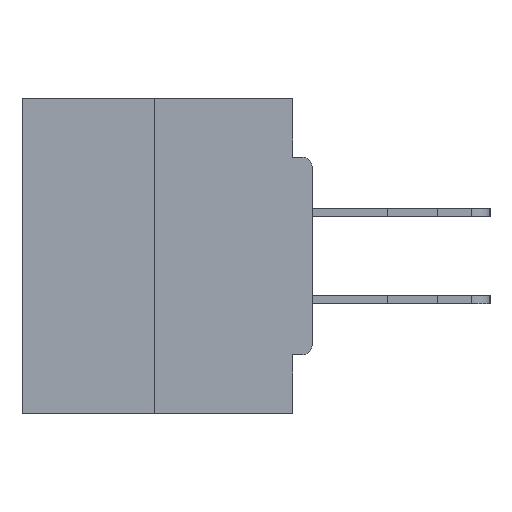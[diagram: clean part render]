
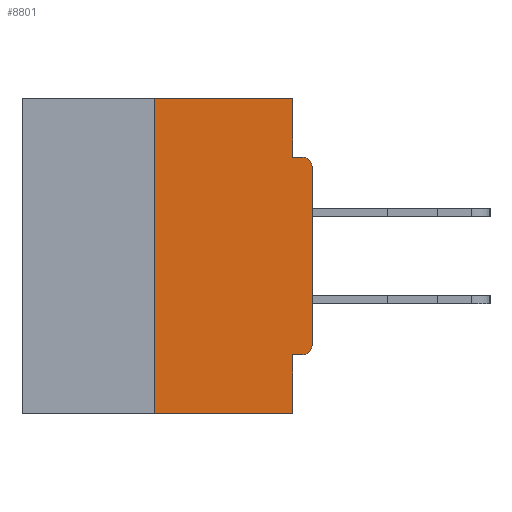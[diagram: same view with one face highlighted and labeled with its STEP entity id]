
A CAD part, left-side view. The second image highlights one B-rep face of the part: STEP entity #8801.
In plain terms, the highlighted planar face has unit normal (-1, 0, 0).
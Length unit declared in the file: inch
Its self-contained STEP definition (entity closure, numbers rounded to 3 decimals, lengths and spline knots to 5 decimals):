
#310 = CARTESIAN_POINT ( 'NONE',  ( 0., 0., -0.1085 ) ) ;
#431 = VERTEX_POINT ( 'NONE', #29109 ) ;
#497 = DIRECTION ( 'NONE',  ( 0., 0., -1. ) ) ;
#1847 = VECTOR ( 'NONE', #18469, 39.37008 ) ;
#2375 = EDGE_LOOP ( 'NONE', ( #6057, #5603, #20990, #12456, #24337, #6280, #20791, #26790, #5908, #17580 ) ) ;
#2600 = PLANE ( 'NONE',  #28627 ) ;
#3042 = VERTEX_POINT ( 'NONE', #310 ) ;
#3046 = EDGE_CURVE ( 'NONE', #3042, #20234, #15409, .T. ) ;
#3607 = DIRECTION ( 'NONE',  ( -1., 0., 0. ) ) ;
#3684 = CARTESIAN_POINT ( 'NONE',  ( 0., 0.015, -0.4065 ) ) ;
#3740 = CARTESIAN_POINT ( 'NONE',  ( 0., 0.46, 0. ) ) ;
#4171 = CARTESIAN_POINT ( 'NONE',  ( 0., 0.031, -0.0935 ) ) ;
#4238 = CARTESIAN_POINT ( 'NONE',  ( 0., 0.25, -0.5 ) ) ;
#4632 = CARTESIAN_POINT ( 'NONE',  ( 0., 0., 0. ) ) ;
#4866 = AXIS2_PLACEMENT_3D ( 'NONE', #27435, #3607, #22065 ) ;
#4919 = VECTOR ( 'NONE', #14685, 39.37008 ) ;
#5404 = EDGE_CURVE ( 'NONE', #27417, #28731, #22710, .T. ) ;
#5603 = ORIENTED_EDGE ( 'NONE', *, *, #30233, .F. ) ;
#5655 = DIRECTION ( 'NONE',  ( 0., -1., 0. ) ) ;
#5908 = ORIENTED_EDGE ( 'NONE', *, *, #34198, .F. ) ;
#6057 = ORIENTED_EDGE ( 'NONE', *, *, #5404, .F. ) ;
#6280 = ORIENTED_EDGE ( 'NONE', *, *, #24998, .T. ) ;
#6614 = DIRECTION ( 'NONE',  ( 0., -1., 0. ) ) ;
#7896 = EDGE_CURVE ( 'NONE', #29916, #29192, #21780, .T. ) ;
#8348 = CARTESIAN_POINT ( 'NONE',  ( 0., 0.25, 0. ) ) ;
#8578 = CIRCLE ( 'NONE', #30166, 0.015 ) ;
#8801 = ADVANCED_FACE ( 'NONE', ( #24159 ), #2600, .F. ) ;
#9552 = DIRECTION ( 'NONE',  ( 0., 0., -1. ) ) ;
#11156 = LINE ( 'NONE', #14273, #20593 ) ;
#12456 = ORIENTED_EDGE ( 'NONE', *, *, #13436, .F. ) ;
#12875 = DIRECTION ( 'NONE',  ( 0., 0., -1. ) ) ;
#13323 = CARTESIAN_POINT ( 'NONE',  ( 0., 0.46, -0.5 ) ) ;
#13436 = EDGE_CURVE ( 'NONE', #29192, #26889, #29585, .T. ) ;
#13791 = VECTOR ( 'NONE', #18961, 39.37008 ) ;
#14104 = VECTOR ( 'NONE', #27179, 39.37008 ) ;
#14273 = CARTESIAN_POINT ( 'NONE',  ( 0., 0., -0.0935 ) ) ;
#14685 = DIRECTION ( 'NONE',  ( 0., -1., 0. ) ) ;
#15240 = DIRECTION ( 'NONE',  ( 0., 0., 1. ) ) ;
#15409 = CIRCLE ( 'NONE', #4866, 0.015 ) ;
#15645 = CARTESIAN_POINT ( 'NONE',  ( 0., 0.46, 0. ) ) ;
#15684 = CARTESIAN_POINT ( 'NONE',  ( 0., 0.031, -0.5 ) ) ;
#16388 = CARTESIAN_POINT ( 'NONE',  ( 0., 0., -0.4065 ) ) ;
#16630 = VECTOR ( 'NONE', #12875, 39.37008 ) ;
#17580 = ORIENTED_EDGE ( 'NONE', *, *, #32826, .F. ) ;
#17658 = VECTOR ( 'NONE', #15240, 39.37008 ) ;
#17843 = EDGE_CURVE ( 'NONE', #21377, #26889, #18893, .T. ) ;
#18469 = DIRECTION ( 'NONE',  ( 0., 0., -1. ) ) ;
#18893 = LINE ( 'NONE', #13323, #19761 ) ;
#18940 = DIRECTION ( 'NONE',  ( 1., 0., 0. ) ) ;
#18961 = DIRECTION ( 'NONE',  ( 0., 0., 1. ) ) ;
#19761 = VECTOR ( 'NONE', #5655, 39.37008 ) ;
#20234 = VERTEX_POINT ( 'NONE', #33246 ) ;
#20593 = VECTOR ( 'NONE', #6614, 39.37008 ) ;
#20791 = ORIENTED_EDGE ( 'NONE', *, *, #30976, .T. ) ;
#20990 = ORIENTED_EDGE ( 'NONE', *, *, #17843, .T. ) ;
#21339 = CARTESIAN_POINT ( 'NONE',  ( 0., 0.031, 0. ) ) ;
#21377 = VERTEX_POINT ( 'NONE', #4238 ) ;
#21780 = LINE ( 'NONE', #16388, #14104 ) ;
#22065 = DIRECTION ( 'NONE',  ( 0., 0., -1. ) ) ;
#22710 = LINE ( 'NONE', #3740, #4919 ) ;
#22786 = CARTESIAN_POINT ( 'NONE',  ( 0., 0.015, -0.3915 ) ) ;
#23662 = CARTESIAN_POINT ( 'NONE',  ( 0., 0.031, 0. ) ) ;
#23735 = CARTESIAN_POINT ( 'NONE',  ( 0., 0.25, 0. ) ) ;
#24159 = FACE_OUTER_BOUND ( 'NONE', #2375, .T. ) ;
#24337 = ORIENTED_EDGE ( 'NONE', *, *, #7896, .F. ) ;
#24976 = VERTEX_POINT ( 'NONE', #4171 ) ;
#24998 = EDGE_CURVE ( 'NONE', #29916, #431, #8578, .T. ) ;
#26445 = LINE ( 'NONE', #23662, #16630 ) ;
#26790 = ORIENTED_EDGE ( 'NONE', *, *, #3046, .T. ) ;
#26889 = VERTEX_POINT ( 'NONE', #26892 ) ;
#26892 = CARTESIAN_POINT ( 'NONE',  ( 0., 0.031, -0.5 ) ) ;
#27179 = DIRECTION ( 'NONE',  ( 0., 1., 0. ) ) ;
#27417 = VERTEX_POINT ( 'NONE', #23735 ) ;
#27435 = CARTESIAN_POINT ( 'NONE',  ( 0., 0.015, -0.1085 ) ) ;
#28292 = CARTESIAN_POINT ( 'NONE',  ( 0., 0.031, -0.4065 ) ) ;
#28627 = AXIS2_PLACEMENT_3D ( 'NONE', #15645, #18940, #497 ) ;
#28731 = VERTEX_POINT ( 'NONE', #21339 ) ;
#29109 = CARTESIAN_POINT ( 'NONE',  ( 0., 0., -0.3915 ) ) ;
#29192 = VERTEX_POINT ( 'NONE', #28292 ) ;
#29585 = LINE ( 'NONE', #15684, #1847 ) ;
#29611 = LINE ( 'NONE', #4632, #17658 ) ;
#29916 = VERTEX_POINT ( 'NONE', #3684 ) ;
#30166 = AXIS2_PLACEMENT_3D ( 'NONE', #22786, #33564, #9552 ) ;
#30233 = EDGE_CURVE ( 'NONE', #21377, #27417, #32857, .T. ) ;
#30976 = EDGE_CURVE ( 'NONE', #431, #3042, #29611, .T. ) ;
#32826 = EDGE_CURVE ( 'NONE', #28731, #24976, #26445, .T. ) ;
#32857 = LINE ( 'NONE', #8348, #13791 ) ;
#33246 = CARTESIAN_POINT ( 'NONE',  ( 0., 0.015, -0.0935 ) ) ;
#33564 = DIRECTION ( 'NONE',  ( -1., 0., 0. ) ) ;
#34198 = EDGE_CURVE ( 'NONE', #24976, #20234, #11156, .T. ) ;
